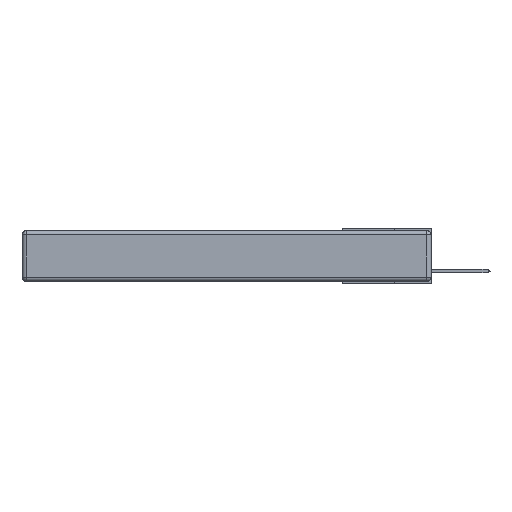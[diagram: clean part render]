
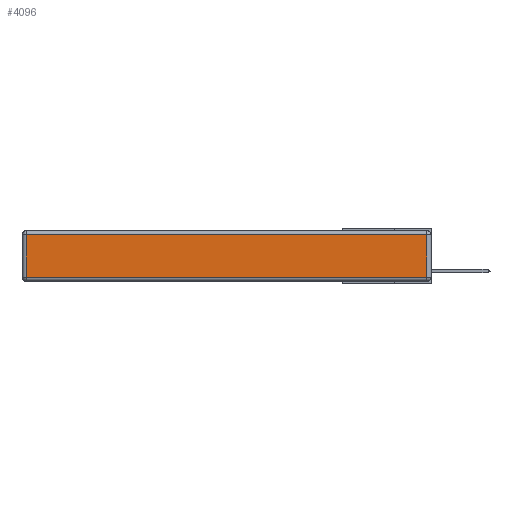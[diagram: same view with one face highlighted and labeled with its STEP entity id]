
A CAD part, left-side view. The second image highlights one B-rep face of the part: STEP entity #4096.
In plain terms, the highlighted planar face has unit normal (-1, 0, 0).
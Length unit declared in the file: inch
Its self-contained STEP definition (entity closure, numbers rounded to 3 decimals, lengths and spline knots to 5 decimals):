
#220 = PLANE ( 'NONE',  #24499 ) ;
#750 = VECTOR ( 'NONE', #17867, 39.37008 ) ;
#2635 = DIRECTION ( 'NONE',  ( 0., 0., 1. ) ) ;
#3278 = DIRECTION ( 'NONE',  ( 0., 0., 1. ) ) ;
#3548 = CARTESIAN_POINT ( 'NONE',  ( 0., 2.75, -0.03 ) ) ;
#4096 = ADVANCED_FACE ( 'NONE', ( #20650 ), #220, .T. ) ;
#5021 = CARTESIAN_POINT ( 'NONE',  ( 0., 2.72, -0.343 ) ) ;
#5718 = CARTESIAN_POINT ( 'NONE',  ( 0., 0., -0.343 ) ) ;
#7826 = CARTESIAN_POINT ( 'NONE',  ( 0., 0.03, -0.313 ) ) ;
#7840 = DIRECTION ( 'NONE',  ( -1., 0., 0. ) ) ;
#8529 = DIRECTION ( 'NONE',  ( 0., 1., 0. ) ) ;
#8699 = VERTEX_POINT ( 'NONE', #7826 ) ;
#9120 = LINE ( 'NONE', #25586, #10669 ) ;
#10618 = CARTESIAN_POINT ( 'NONE',  ( 0., 2.72, -0.03 ) ) ;
#10669 = VECTOR ( 'NONE', #3278, 39.37008 ) ;
#12184 = VERTEX_POINT ( 'NONE', #15179 ) ;
#13798 = VERTEX_POINT ( 'NONE', #26201 ) ;
#15179 = CARTESIAN_POINT ( 'NONE',  ( 0., 0.03, -0.03 ) ) ;
#15488 = LINE ( 'NONE', #5021, #750 ) ;
#16132 = LINE ( 'NONE', #3548, #23510 ) ;
#17867 = DIRECTION ( 'NONE',  ( 0., 0., -1. ) ) ;
#18453 = ORIENTED_EDGE ( 'NONE', *, *, #26414, .T. ) ;
#20650 = FACE_OUTER_BOUND ( 'NONE', #27421, .T. ) ;
#21580 = ORIENTED_EDGE ( 'NONE', *, *, #21941, .T. ) ;
#21941 = EDGE_CURVE ( 'NONE', #8699, #12184, #9120, .T. ) ;
#21978 = VERTEX_POINT ( 'NONE', #10618 ) ;
#22632 = DIRECTION ( 'NONE',  ( 0., -1., 0. ) ) ;
#23253 = EDGE_CURVE ( 'NONE', #13798, #8699, #28132, .T. ) ;
#23510 = VECTOR ( 'NONE', #8529, 39.37008 ) ;
#24499 = AXIS2_PLACEMENT_3D ( 'NONE', #5718, #7840, #2635 ) ;
#24985 = VECTOR ( 'NONE', #22632, 39.37008 ) ;
#25586 = CARTESIAN_POINT ( 'NONE',  ( 0., 0.03, -0.343 ) ) ;
#26201 = CARTESIAN_POINT ( 'NONE',  ( 0., 2.72, -0.313 ) ) ;
#26414 = EDGE_CURVE ( 'NONE', #21978, #13798, #15488, .T. ) ;
#27421 = EDGE_LOOP ( 'NONE', ( #28276, #21580, #28240, #18453 ) ) ;
#28132 = LINE ( 'NONE', #29922, #24985 ) ;
#28240 = ORIENTED_EDGE ( 'NONE', *, *, #28424, .T. ) ;
#28276 = ORIENTED_EDGE ( 'NONE', *, *, #23253, .T. ) ;
#28424 = EDGE_CURVE ( 'NONE', #12184, #21978, #16132, .T. ) ;
#29922 = CARTESIAN_POINT ( 'NONE',  ( 0., 0., -0.313 ) ) ;
